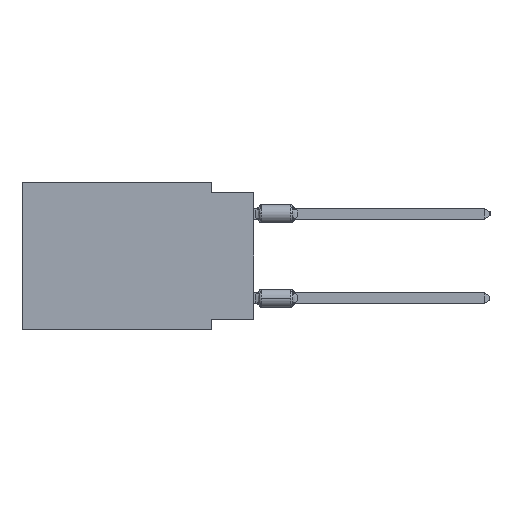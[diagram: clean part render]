
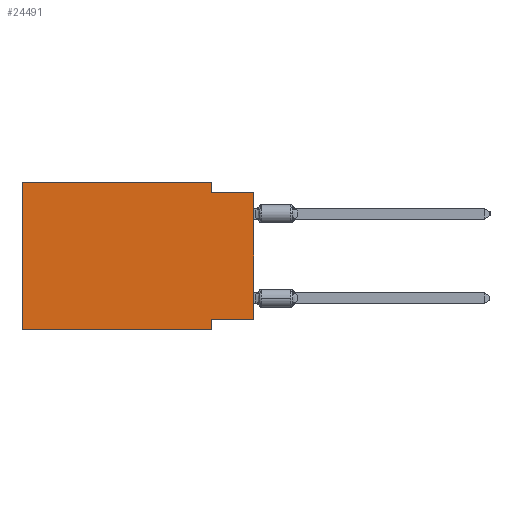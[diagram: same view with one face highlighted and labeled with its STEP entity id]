
A CAD part, left-side view. The second image highlights one B-rep face of the part: STEP entity #24491.
In plain terms, the highlighted planar face has unit normal (-1, 0, 0).
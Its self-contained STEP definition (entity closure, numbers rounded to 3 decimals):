
#2191 = LINE ( 'NONE', #42386, #35529 ) ;
#5928 = EDGE_CURVE ( 'NONE', #20422, #49015, #36684, .T. ) ;
#6223 = VECTOR ( 'NONE', #39916, 1000. ) ;
#7998 = DIRECTION ( 'NONE',  ( 0., 0., -1. ) ) ;
#9584 = ORIENTED_EDGE ( 'NONE', *, *, #16971, .F. ) ;
#10029 = DIRECTION ( 'NONE',  ( 0., 0., -1. ) ) ;
#11740 = CARTESIAN_POINT ( 'NONE',  ( 0., 2.54, -8.89 ) ) ;
#13127 = EDGE_CURVE ( 'NONE', #18964, #21414, #15165, .T. ) ;
#13343 = CARTESIAN_POINT ( 'NONE',  ( 0., 2.54, -0.635 ) ) ;
#13530 = CARTESIAN_POINT ( 'NONE',  ( 0., 0., -0.635 ) ) ;
#13587 = ORIENTED_EDGE ( 'NONE', *, *, #31576, .T. ) ;
#13688 = CARTESIAN_POINT ( 'NONE',  ( 0., 13.97, -8.89 ) ) ;
#14151 = LINE ( 'NONE', #32235, #38685 ) ;
#15165 = LINE ( 'NONE', #45867, #18752 ) ;
#15617 = LINE ( 'NONE', #55793, #17484 ) ;
#16101 = VECTOR ( 'NONE', #20516, 1000. ) ;
#16971 = EDGE_CURVE ( 'NONE', #49015, #21414, #17538, .T. ) ;
#17484 = VECTOR ( 'NONE', #33410, 1000. ) ;
#17538 = LINE ( 'NONE', #13530, #6223 ) ;
#18512 = ORIENTED_EDGE ( 'NONE', *, *, #20716, .F. ) ;
#18752 = VECTOR ( 'NONE', #54761, 1000. ) ;
#18964 = VERTEX_POINT ( 'NONE', #23916 ) ;
#20003 = EDGE_CURVE ( 'NONE', #30327, #23077, #55344, .T. ) ;
#20422 = VERTEX_POINT ( 'NONE', #33481 ) ;
#20516 = DIRECTION ( 'NONE',  ( 0., -1., 0. ) ) ;
#20716 = EDGE_CURVE ( 'NONE', #18964, #30327, #15617, .T. ) ;
#20904 = EDGE_LOOP ( 'NONE', ( #46023, #9584, #56118, #43698, #21838, #13587, #52335, #18512 ) ) ;
#21414 = VERTEX_POINT ( 'NONE', #25629 ) ;
#21838 = ORIENTED_EDGE ( 'NONE', *, *, #37901, .F. ) ;
#23077 = VERTEX_POINT ( 'NONE', #39785 ) ;
#23916 = CARTESIAN_POINT ( 'NONE',  ( 0., 0., -8.255 ) ) ;
#24260 = CARTESIAN_POINT ( 'NONE',  ( 0., 13.97, 0. ) ) ;
#24491 = ADVANCED_FACE ( 'NONE', ( #35567 ), #53061, .F. ) ;
#25629 = CARTESIAN_POINT ( 'NONE',  ( 0., 0., -0.635 ) ) ;
#26528 = VECTOR ( 'NONE', #41275, 1000. ) ;
#27249 = CARTESIAN_POINT ( 'NONE',  ( 0., 13.97, 0. ) ) ;
#28656 = EDGE_CURVE ( 'NONE', #54923, #20422, #42915, .T. ) ;
#28824 = AXIS2_PLACEMENT_3D ( 'NONE', #27249, #53642, #10029 ) ;
#30327 = VERTEX_POINT ( 'NONE', #39395 ) ;
#31576 = EDGE_CURVE ( 'NONE', #49842, #23077, #2191, .T. ) ;
#32235 = CARTESIAN_POINT ( 'NONE',  ( 0., 13.97, 0. ) ) ;
#32386 = CARTESIAN_POINT ( 'NONE',  ( 0., 2.54, 0. ) ) ;
#33410 = DIRECTION ( 'NONE',  ( 0., 1., 0. ) ) ;
#33481 = CARTESIAN_POINT ( 'NONE',  ( 0., 2.54, 0. ) ) ;
#33494 = DIRECTION ( 'NONE',  ( 0., -1., 0. ) ) ;
#35529 = VECTOR ( 'NONE', #33494, 1000. ) ;
#35567 = FACE_OUTER_BOUND ( 'NONE', #20904, .T. ) ;
#36539 = DIRECTION ( 'NONE',  ( 0., 0., 1. ) ) ;
#36684 = LINE ( 'NONE', #32386, #26528 ) ;
#37901 = EDGE_CURVE ( 'NONE', #49842, #54923, #14151, .T. ) ;
#38685 = VECTOR ( 'NONE', #36539, 1000. ) ;
#39395 = CARTESIAN_POINT ( 'NONE',  ( 0., 2.54, -8.255 ) ) ;
#39785 = CARTESIAN_POINT ( 'NONE',  ( 0., 2.54, -8.89 ) ) ;
#39916 = DIRECTION ( 'NONE',  ( 0., -1., 0. ) ) ;
#41275 = DIRECTION ( 'NONE',  ( 0., 0., -1. ) ) ;
#42386 = CARTESIAN_POINT ( 'NONE',  ( 0., 13.97, -8.89 ) ) ;
#42915 = LINE ( 'NONE', #24260, #16101 ) ;
#43698 = ORIENTED_EDGE ( 'NONE', *, *, #28656, .F. ) ;
#45867 = CARTESIAN_POINT ( 'NONE',  ( 0., 0., 0. ) ) ;
#46023 = ORIENTED_EDGE ( 'NONE', *, *, #13127, .T. ) ;
#49015 = VERTEX_POINT ( 'NONE', #13343 ) ;
#49842 = VERTEX_POINT ( 'NONE', #13688 ) ;
#51627 = CARTESIAN_POINT ( 'NONE',  ( 0., 13.97, 0. ) ) ;
#52335 = ORIENTED_EDGE ( 'NONE', *, *, #20003, .F. ) ;
#53061 = PLANE ( 'NONE',  #28824 ) ;
#53642 = DIRECTION ( 'NONE',  ( 1., 0., 0. ) ) ;
#54761 = DIRECTION ( 'NONE',  ( 0., 0., 1. ) ) ;
#54923 = VERTEX_POINT ( 'NONE', #51627 ) ;
#55037 = VECTOR ( 'NONE', #7998, 1000. ) ;
#55344 = LINE ( 'NONE', #11740, #55037 ) ;
#55793 = CARTESIAN_POINT ( 'NONE',  ( 0., 0., -8.255 ) ) ;
#56118 = ORIENTED_EDGE ( 'NONE', *, *, #5928, .F. ) ;
